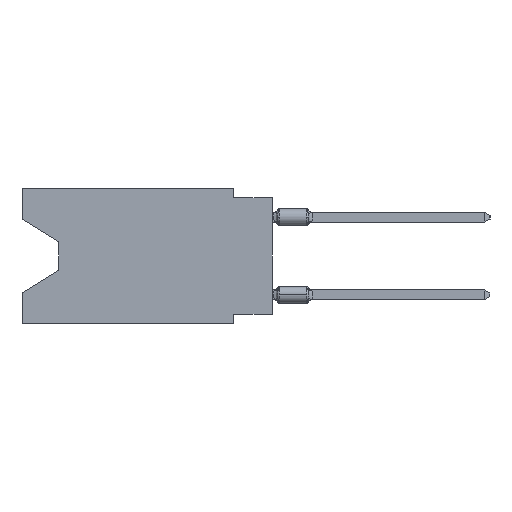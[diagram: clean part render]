
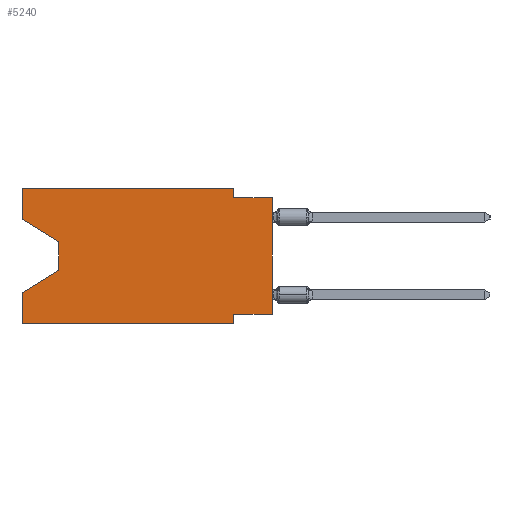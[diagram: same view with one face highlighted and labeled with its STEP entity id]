
A CAD part, left-side view. The second image highlights one B-rep face of the part: STEP entity #5240.
In plain terms, the highlighted planar face has unit normal (-1, 0, 0).
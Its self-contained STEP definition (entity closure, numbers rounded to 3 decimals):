
#36 = EDGE_CURVE ( 'NONE', #6188, #23949, #7539, .T. ) ;
#250 = VECTOR ( 'NONE', #9019, 1000. ) ;
#718 = ORIENTED_EDGE ( 'NONE', *, *, #22490, .T. ) ;
#1301 = VERTEX_POINT ( 'NONE', #41167 ) ;
#1351 = ORIENTED_EDGE ( 'NONE', *, *, #7634, .F. ) ;
#1354 = VERTEX_POINT ( 'NONE', #40158 ) ;
#1556 = CARTESIAN_POINT ( 'NONE',  ( 0., 16.383, 0. ) ) ;
#2004 = VECTOR ( 'NONE', #16997, 1000. ) ;
#3058 = VECTOR ( 'NONE', #40292, 1000. ) ;
#3208 = FACE_OUTER_BOUND ( 'NONE', #39638, .T. ) ;
#3556 = CARTESIAN_POINT ( 'NONE',  ( 0., 16.383, -6.852 ) ) ;
#4531 = ORIENTED_EDGE ( 'NONE', *, *, #29719, .T. ) ;
#4558 = DIRECTION ( 'NONE',  ( 0., 0.855, -0.519 ) ) ;
#4831 = ORIENTED_EDGE ( 'NONE', *, *, #36, .T. ) ;
#4940 = VECTOR ( 'NONE', #4558, 1000. ) ;
#5240 = ADVANCED_FACE ( 'NONE', ( #3208 ), #18970, .F. ) ;
#5807 = EDGE_CURVE ( 'NONE', #1354, #33689, #36373, .T. ) ;
#6016 = EDGE_CURVE ( 'NONE', #30484, #12455, #15100, .T. ) ;
#6188 = VERTEX_POINT ( 'NONE', #19133 ) ;
#7539 = LINE ( 'NONE', #26928, #4940 ) ;
#7543 = ORIENTED_EDGE ( 'NONE', *, *, #40434, .F. ) ;
#7634 = EDGE_CURVE ( 'NONE', #22161, #1301, #16815, .T. ) ;
#8784 = ORIENTED_EDGE ( 'NONE', *, *, #40455, .F. ) ;
#9019 = DIRECTION ( 'NONE',  ( 0., 0., 1. ) ) ;
#9199 = VERTEX_POINT ( 'NONE', #15328 ) ;
#9401 = CARTESIAN_POINT ( 'NONE',  ( 0., 16.383, 0. ) ) ;
#9449 = CARTESIAN_POINT ( 'NONE',  ( 0., 2.54, -8.89 ) ) ;
#10340 = VERTEX_POINT ( 'NONE', #20892 ) ;
#10605 = LINE ( 'NONE', #14453, #15667 ) ;
#10933 = DIRECTION ( 'NONE',  ( 0., 0., 1. ) ) ;
#11037 = DIRECTION ( 'NONE',  ( 0., 0., -1. ) ) ;
#11592 = ORIENTED_EDGE ( 'NONE', *, *, #5807, .F. ) ;
#12002 = VECTOR ( 'NONE', #35313, 1000. ) ;
#12146 = DIRECTION ( 'NONE',  ( 0., 0., -1. ) ) ;
#12440 = LINE ( 'NONE', #35191, #250 ) ;
#12455 = VERTEX_POINT ( 'NONE', #9449 ) ;
#12509 = VECTOR ( 'NONE', #12146, 1000. ) ;
#13006 = DIRECTION ( 'NONE',  ( 0., -1., 0. ) ) ;
#13101 = VECTOR ( 'NONE', #30207, 1000. ) ;
#13511 = CARTESIAN_POINT ( 'NONE',  ( 0., 16.383, -2.038 ) ) ;
#14453 = CARTESIAN_POINT ( 'NONE',  ( 0., 2.54, 0. ) ) ;
#15100 = LINE ( 'NONE', #18083, #29417 ) ;
#15328 = CARTESIAN_POINT ( 'NONE',  ( 0., 2.54, -0.635 ) ) ;
#15417 = VECTOR ( 'NONE', #13006, 1000. ) ;
#15667 = VECTOR ( 'NONE', #11037, 1000. ) ;
#16815 = LINE ( 'NONE', #39344, #15417 ) ;
#16997 = DIRECTION ( 'NONE',  ( 0., 0., -1. ) ) ;
#17283 = CARTESIAN_POINT ( 'NONE',  ( 0., 16.383, -2.038 ) ) ;
#18083 = CARTESIAN_POINT ( 'NONE',  ( 0., 16.383, -8.89 ) ) ;
#18411 = EDGE_CURVE ( 'NONE', #1301, #9199, #10605, .T. ) ;
#18970 = PLANE ( 'NONE',  #19166 ) ;
#19133 = CARTESIAN_POINT ( 'NONE',  ( 0., 13.97, -5.385 ) ) ;
#19166 = AXIS2_PLACEMENT_3D ( 'NONE', #9401, #35342, #20002 ) ;
#20002 = DIRECTION ( 'NONE',  ( 0., 0., -1. ) ) ;
#20027 = ORIENTED_EDGE ( 'NONE', *, *, #6016, .T. ) ;
#20892 = CARTESIAN_POINT ( 'NONE',  ( 0., 13.97, -3.505 ) ) ;
#21151 = LINE ( 'NONE', #1556, #21404 ) ;
#21404 = VECTOR ( 'NONE', #10933, 1000. ) ;
#21966 = VECTOR ( 'NONE', #30243, 1000. ) ;
#22161 = VERTEX_POINT ( 'NONE', #31170 ) ;
#22348 = CARTESIAN_POINT ( 'NONE',  ( 0., 0., -0.635 ) ) ;
#22490 = EDGE_CURVE ( 'NONE', #10340, #6188, #34678, .T. ) ;
#22673 = EDGE_CURVE ( 'NONE', #33689, #12455, #29562, .T. ) ;
#22877 = ORIENTED_EDGE ( 'NONE', *, *, #28211, .T. ) ;
#23230 = LINE ( 'NONE', #17283, #21966 ) ;
#23930 = LINE ( 'NONE', #36889, #3058 ) ;
#23949 = VERTEX_POINT ( 'NONE', #3556 ) ;
#24745 = ORIENTED_EDGE ( 'NONE', *, *, #35235, .F. ) ;
#26928 = CARTESIAN_POINT ( 'NONE',  ( 0., 13.97, -5.385 ) ) ;
#27020 = CARTESIAN_POINT ( 'NONE',  ( 0., 0., -8.255 ) ) ;
#28211 = EDGE_CURVE ( 'NONE', #38988, #10340, #23230, .T. ) ;
#28447 = ORIENTED_EDGE ( 'NONE', *, *, #22673, .F. ) ;
#29417 = VECTOR ( 'NONE', #37210, 1000. ) ;
#29562 = LINE ( 'NONE', #29962, #2004 ) ;
#29719 = EDGE_CURVE ( 'NONE', #1354, #32294, #12440, .T. ) ;
#29962 = CARTESIAN_POINT ( 'NONE',  ( 0., 2.54, -8.89 ) ) ;
#30207 = DIRECTION ( 'NONE',  ( 0., 1., 0. ) ) ;
#30243 = DIRECTION ( 'NONE',  ( 0., -0.855, -0.519 ) ) ;
#30484 = VERTEX_POINT ( 'NONE', #38225 ) ;
#30576 = CARTESIAN_POINT ( 'NONE',  ( 0., 2.54, -8.255 ) ) ;
#31170 = CARTESIAN_POINT ( 'NONE',  ( 0., 16.383, 0. ) ) ;
#32294 = VERTEX_POINT ( 'NONE', #37662 ) ;
#32354 = LINE ( 'NONE', #22348, #12002 ) ;
#33321 = ORIENTED_EDGE ( 'NONE', *, *, #18411, .F. ) ;
#33689 = VERTEX_POINT ( 'NONE', #30576 ) ;
#34678 = LINE ( 'NONE', #41273, #12509 ) ;
#35191 = CARTESIAN_POINT ( 'NONE',  ( 0., 0., 0. ) ) ;
#35235 = EDGE_CURVE ( 'NONE', #9199, #32294, #32354, .T. ) ;
#35313 = DIRECTION ( 'NONE',  ( 0., -1., 0. ) ) ;
#35342 = DIRECTION ( 'NONE',  ( 1., 0., 0. ) ) ;
#36373 = LINE ( 'NONE', #27020, #13101 ) ;
#36889 = CARTESIAN_POINT ( 'NONE',  ( 0., 16.383, 0. ) ) ;
#37210 = DIRECTION ( 'NONE',  ( 0., -1., 0. ) ) ;
#37662 = CARTESIAN_POINT ( 'NONE',  ( 0., 0., -0.635 ) ) ;
#38225 = CARTESIAN_POINT ( 'NONE',  ( 0., 16.383, -8.89 ) ) ;
#38988 = VERTEX_POINT ( 'NONE', #13511 ) ;
#39344 = CARTESIAN_POINT ( 'NONE',  ( 0., 16.383, 0. ) ) ;
#39638 = EDGE_LOOP ( 'NONE', ( #22877, #718, #4831, #8784, #20027, #28447, #11592, #4531, #24745, #33321, #1351, #7543 ) ) ;
#40158 = CARTESIAN_POINT ( 'NONE',  ( 0., 0., -8.255 ) ) ;
#40292 = DIRECTION ( 'NONE',  ( 0., 0., 1. ) ) ;
#40434 = EDGE_CURVE ( 'NONE', #38988, #22161, #21151, .T. ) ;
#40455 = EDGE_CURVE ( 'NONE', #30484, #23949, #23930, .T. ) ;
#41167 = CARTESIAN_POINT ( 'NONE',  ( 0., 2.54, 0. ) ) ;
#41273 = CARTESIAN_POINT ( 'NONE',  ( 0., 13.97, -3.505 ) ) ;
